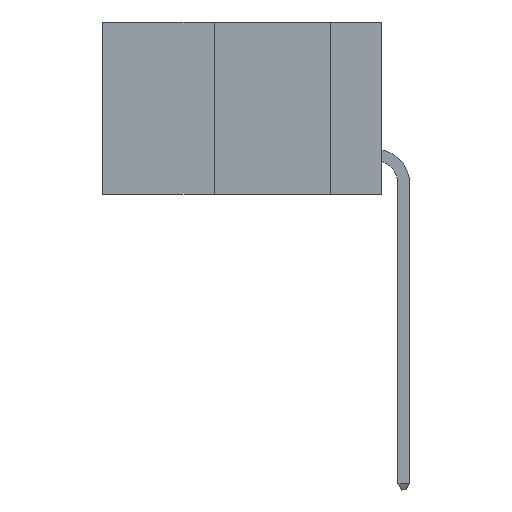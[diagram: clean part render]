
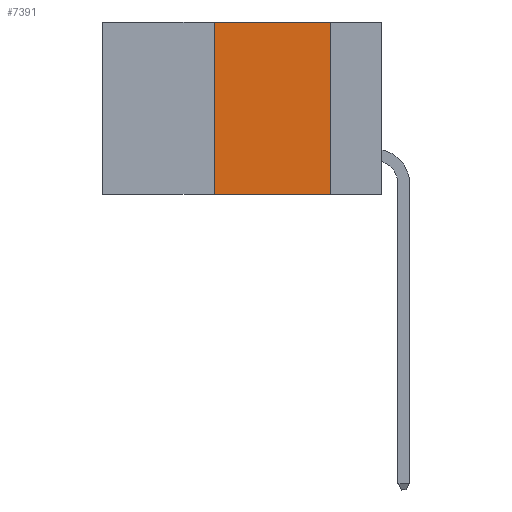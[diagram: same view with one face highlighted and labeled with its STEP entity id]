
A CAD part, left-side view. The second image highlights one B-rep face of the part: STEP entity #7391.
In plain terms, the highlighted planar face has unit normal (-1, 0, 0).
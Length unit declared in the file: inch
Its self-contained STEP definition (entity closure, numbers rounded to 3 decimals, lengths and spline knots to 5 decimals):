
#53 = DIRECTION ( 'NONE',  ( 0., -1., 0. ) ) ;
#160 = DIRECTION ( 'NONE',  ( 0., -1., 0. ) ) ;
#1511 = VERTEX_POINT ( 'NONE', #5440 ) ;
#1589 = FACE_OUTER_BOUND ( 'NONE', #2635, .T. ) ;
#2065 = VECTOR ( 'NONE', #14697, 39.37008 ) ;
#2349 = EDGE_CURVE ( 'NONE', #5158, #2535, #18814, .T. ) ;
#2535 = VERTEX_POINT ( 'NONE', #15573 ) ;
#2635 = EDGE_LOOP ( 'NONE', ( #3482, #13984, #18626, #9497 ) ) ;
#3482 = ORIENTED_EDGE ( 'NONE', *, *, #2349, .F. ) ;
#5158 = VERTEX_POINT ( 'NONE', #14977 ) ;
#5440 = CARTESIAN_POINT ( 'NONE',  ( 0., 0.36, -0.37 ) ) ;
#5481 = CARTESIAN_POINT ( 'NONE',  ( 0., 0.36, 0. ) ) ;
#5877 = DIRECTION ( 'NONE',  ( 0., 0., 1. ) ) ;
#6875 = AXIS2_PLACEMENT_3D ( 'NONE', #16701, #10448, #11978 ) ;
#7193 = VERTEX_POINT ( 'NONE', #5481 ) ;
#7320 = PLANE ( 'NONE',  #6875 ) ;
#7391 = ADVANCED_FACE ( 'NONE', ( #1589 ), #7320, .F. ) ;
#9301 = VECTOR ( 'NONE', #160, 39.37008 ) ;
#9307 = CARTESIAN_POINT ( 'NONE',  ( 0., 0.6, 0. ) ) ;
#9497 = ORIENTED_EDGE ( 'NONE', *, *, #14364, .T. ) ;
#9951 = LINE ( 'NONE', #9307, #16538 ) ;
#10314 = CARTESIAN_POINT ( 'NONE',  ( 0., 0.36, 0. ) ) ;
#10448 = DIRECTION ( 'NONE',  ( 1., 0., 0. ) ) ;
#10880 = CARTESIAN_POINT ( 'NONE',  ( 0., 0.6, -0.37 ) ) ;
#11712 = LINE ( 'NONE', #10880, #9301 ) ;
#11978 = DIRECTION ( 'NONE',  ( 0., 0., -1. ) ) ;
#13556 = VECTOR ( 'NONE', #5877, 39.37008 ) ;
#13984 = ORIENTED_EDGE ( 'NONE', *, *, #15478, .F. ) ;
#14364 = EDGE_CURVE ( 'NONE', #1511, #2535, #11712, .T. ) ;
#14537 = LINE ( 'NONE', #10314, #13556 ) ;
#14697 = DIRECTION ( 'NONE',  ( 0., 0., -1. ) ) ;
#14977 = CARTESIAN_POINT ( 'NONE',  ( 0., 0.11, 0. ) ) ;
#15478 = EDGE_CURVE ( 'NONE', #7193, #5158, #9951, .T. ) ;
#15573 = CARTESIAN_POINT ( 'NONE',  ( 0., 0.11, -0.37 ) ) ;
#16538 = VECTOR ( 'NONE', #53, 39.37008 ) ;
#16701 = CARTESIAN_POINT ( 'NONE',  ( 0., 0.6, 0. ) ) ;
#17789 = CARTESIAN_POINT ( 'NONE',  ( 0., 0.11, 0. ) ) ;
#18626 = ORIENTED_EDGE ( 'NONE', *, *, #19589, .F. ) ;
#18814 = LINE ( 'NONE', #17789, #2065 ) ;
#19589 = EDGE_CURVE ( 'NONE', #1511, #7193, #14537, .T. ) ;
